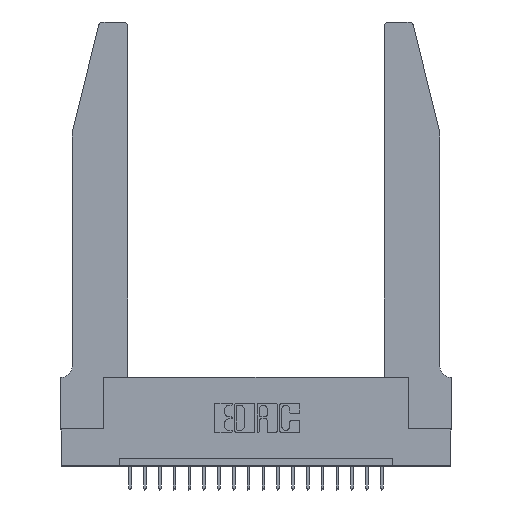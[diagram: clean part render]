
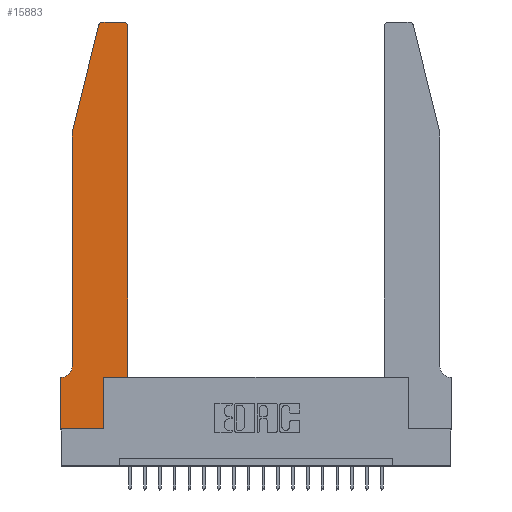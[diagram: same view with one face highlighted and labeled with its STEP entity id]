
A CAD part, top view. The second image highlights one B-rep face of the part: STEP entity #15883.
In plain terms, the highlighted planar face has unit normal (0, 0, 1).
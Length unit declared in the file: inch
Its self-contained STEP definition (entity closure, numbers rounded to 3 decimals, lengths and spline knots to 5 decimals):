
#17 = VECTOR ( 'NONE', #19088, 39.37008 ) ;
#201 = DIRECTION ( 'NONE',  ( -1., 0., 0. ) ) ;
#575 = ORIENTED_EDGE ( 'NONE', *, *, #8515, .T. ) ;
#639 = CARTESIAN_POINT ( 'NONE',  ( 0.4205, 2.75, 0.37 ) ) ;
#790 = DIRECTION ( 'NONE',  ( 0., 1., 0. ) ) ;
#1388 = EDGE_CURVE ( 'NONE', #5708, #19935, #13388, .T. ) ;
#1568 = ORIENTED_EDGE ( 'NONE', *, *, #12442, .T. ) ;
#1596 = DIRECTION ( 'NONE',  ( 1., 0., 0. ) ) ;
#1739 = DIRECTION ( 'NONE',  ( 1., 0., 0. ) ) ;
#1808 = EDGE_CURVE ( 'NONE', #3204, #11223, #20917, .T. ) ;
#1840 = EDGE_CURVE ( 'NONE', #6400, #2131, #21188, .T. ) ;
#1881 = EDGE_CURVE ( 'NONE', #11223, #20557, #5774, .T. ) ;
#1903 = VECTOR ( 'NONE', #7939, 39.37008 ) ;
#2131 = VERTEX_POINT ( 'NONE', #10437 ) ;
#2134 = DIRECTION ( 'NONE',  ( 1., 0., 0. ) ) ;
#2150 = CARTESIAN_POINT ( 'NONE',  ( 0.2865, 0.35, 0.37 ) ) ;
#2797 = VECTOR ( 'NONE', #13358, 39.37008 ) ;
#2940 = LINE ( 'NONE', #2150, #15995 ) ;
#2977 = ORIENTED_EDGE ( 'NONE', *, *, #1881, .T. ) ;
#3045 = ORIENTED_EDGE ( 'NONE', *, *, #10656, .T. ) ;
#3204 = VERTEX_POINT ( 'NONE', #639 ) ;
#3388 = LINE ( 'NONE', #4214, #17 ) ;
#3402 = ORIENTED_EDGE ( 'NONE', *, *, #15248, .T. ) ;
#3446 = ORIENTED_EDGE ( 'NONE', *, *, #16910, .T. ) ;
#3575 = CARTESIAN_POINT ( 'NONE',  ( 0.0755, 2., 0.37 ) ) ;
#3638 = DIRECTION ( 'NONE',  ( -1., 0., 0. ) ) ;
#3684 = CARTESIAN_POINT ( 'NONE',  ( 0.284, 2.72, 0.37 ) ) ;
#3869 = CARTESIAN_POINT ( 'NONE',  ( 0.0055, 0.35, 0.37 ) ) ;
#3877 = DIRECTION ( 'NONE',  ( 0., 0., 1. ) ) ;
#4214 = CARTESIAN_POINT ( 'NONE',  ( 0.4505, 0.35, 0.37 ) ) ;
#4761 = DIRECTION ( 'NONE',  ( 1., 0., 0. ) ) ;
#5011 = DIRECTION ( 'NONE',  ( -1., 0., 0. ) ) ;
#5015 = CARTESIAN_POINT ( 'NONE',  ( 0.0755, 2., 0.37 ) ) ;
#5204 = CARTESIAN_POINT ( 'NONE',  ( 0.4505, 2.72, 0.37 ) ) ;
#5616 = CIRCLE ( 'NONE', #18930, 0.03 ) ;
#5708 = VERTEX_POINT ( 'NONE', #9108 ) ;
#5774 = CIRCLE ( 'NONE', #16114, 0.03 ) ;
#6172 = EDGE_CURVE ( 'NONE', #19386, #3204, #5616, .T. ) ;
#6400 = VERTEX_POINT ( 'NONE', #20015 ) ;
#6699 = CARTESIAN_POINT ( 'NONE',  ( 0., 0., 0.37 ) ) ;
#6913 = CARTESIAN_POINT ( 'NONE',  ( 0.25487, 2.72718, 0.37 ) ) ;
#7939 = DIRECTION ( 'NONE',  ( -0.239, -0.971, 0. ) ) ;
#8505 = ORIENTED_EDGE ( 'NONE', *, *, #19417, .T. ) ;
#8515 = EDGE_CURVE ( 'NONE', #15281, #6400, #2940, .T. ) ;
#8684 = ORIENTED_EDGE ( 'NONE', *, *, #1388, .T. ) ;
#8704 = CARTESIAN_POINT ( 'NONE',  ( 0.0755, 0.35, 0.37 ) ) ;
#8760 = CARTESIAN_POINT ( 'NONE',  ( 0.4205, 2.72, 0.37 ) ) ;
#8898 = DIRECTION ( 'NONE',  ( 0., 0., -1. ) ) ;
#9108 = CARTESIAN_POINT ( 'NONE',  ( 0.0755, 0.42, 0.37 ) ) ;
#9247 = VERTEX_POINT ( 'NONE', #16477 ) ;
#9501 = DIRECTION ( 'NONE',  ( 0., 0., 1. ) ) ;
#9947 = VECTOR ( 'NONE', #5011, 39.37008 ) ;
#10172 = AXIS2_PLACEMENT_3D ( 'NONE', #13110, #9501, #4761 ) ;
#10437 = CARTESIAN_POINT ( 'NONE',  ( 0.4505, 0.35, 0.37 ) ) ;
#10559 = FACE_OUTER_BOUND ( 'NONE', #17041, .T. ) ;
#10656 = EDGE_CURVE ( 'NONE', #2131, #19386, #3388, .T. ) ;
#11223 = VERTEX_POINT ( 'NONE', #12341 ) ;
#11226 = CARTESIAN_POINT ( 'NONE',  ( 0.2865, 0., 0.37 ) ) ;
#12341 = CARTESIAN_POINT ( 'NONE',  ( 0.284, 2.75, 0.37 ) ) ;
#12442 = EDGE_CURVE ( 'NONE', #9247, #15281, #13769, .T. ) ;
#12473 = AXIS2_PLACEMENT_3D ( 'NONE', #15330, #8898, #3638 ) ;
#12621 = CARTESIAN_POINT ( 'NONE',  ( 0.0755, 2., 0.37 ) ) ;
#12951 = LINE ( 'NONE', #12621, #16333 ) ;
#12958 = CARTESIAN_POINT ( 'NONE',  ( 0., 0., 0.37 ) ) ;
#13110 = CARTESIAN_POINT ( 'NONE',  ( 0., 0.35, 0.37 ) ) ;
#13222 = CARTESIAN_POINT ( 'NONE',  ( 0.4505, 0.35, 0.37 ) ) ;
#13358 = DIRECTION ( 'NONE',  ( 0., -1., 0. ) ) ;
#13388 = CIRCLE ( 'NONE', #12473, 0.07 ) ;
#13651 = ORIENTED_EDGE ( 'NONE', *, *, #1840, .T. ) ;
#13769 = LINE ( 'NONE', #12958, #14058 ) ;
#14039 = LINE ( 'NONE', #6699, #2797 ) ;
#14058 = VECTOR ( 'NONE', #21166, 39.37008 ) ;
#14067 = ORIENTED_EDGE ( 'NONE', *, *, #20457, .T. ) ;
#14738 = LINE ( 'NONE', #3575, #1903 ) ;
#15042 = CARTESIAN_POINT ( 'NONE',  ( 0.2605, 2.75, 0.37 ) ) ;
#15169 = DIRECTION ( 'NONE',  ( 0., 0., 1. ) ) ;
#15248 = EDGE_CURVE ( 'NONE', #18689, #5708, #12951, .T. ) ;
#15281 = VERTEX_POINT ( 'NONE', #11226 ) ;
#15330 = CARTESIAN_POINT ( 'NONE',  ( 0.0055, 0.42, 0.37 ) ) ;
#15602 = ORIENTED_EDGE ( 'NONE', *, *, #1808, .T. ) ;
#15883 = ADVANCED_FACE ( 'NONE', ( #10559 ), #21183, .T. ) ;
#15995 = VECTOR ( 'NONE', #790, 39.37008 ) ;
#16114 = AXIS2_PLACEMENT_3D ( 'NONE', #3684, #15169, #1739 ) ;
#16333 = VECTOR ( 'NONE', #20777, 39.37008 ) ;
#16477 = CARTESIAN_POINT ( 'NONE',  ( 0., 0., 0.37 ) ) ;
#16761 = VECTOR ( 'NONE', #1596, 39.37008 ) ;
#16910 = EDGE_CURVE ( 'NONE', #20557, #18689, #14738, .T. ) ;
#17041 = EDGE_LOOP ( 'NONE', ( #15602, #2977, #3446, #3402, #8684, #8505, #14067, #1568, #575, #13651, #3045, #18077 ) ) ;
#18077 = ORIENTED_EDGE ( 'NONE', *, *, #6172, .T. ) ;
#18689 = VERTEX_POINT ( 'NONE', #5015 ) ;
#18744 = LINE ( 'NONE', #8704, #21626 ) ;
#18930 = AXIS2_PLACEMENT_3D ( 'NONE', #8760, #3877, #2134 ) ;
#18964 = CARTESIAN_POINT ( 'NONE',  ( 0., 0.35, 0.37 ) ) ;
#19088 = DIRECTION ( 'NONE',  ( 0., 1., 0. ) ) ;
#19386 = VERTEX_POINT ( 'NONE', #5204 ) ;
#19417 = EDGE_CURVE ( 'NONE', #19935, #20054, #18744, .T. ) ;
#19935 = VERTEX_POINT ( 'NONE', #3869 ) ;
#20015 = CARTESIAN_POINT ( 'NONE',  ( 0.2865, 0.35, 0.37 ) ) ;
#20054 = VERTEX_POINT ( 'NONE', #18964 ) ;
#20457 = EDGE_CURVE ( 'NONE', #20054, #9247, #14039, .T. ) ;
#20557 = VERTEX_POINT ( 'NONE', #6913 ) ;
#20777 = DIRECTION ( 'NONE',  ( 0., -1., 0. ) ) ;
#20917 = LINE ( 'NONE', #15042, #9947 ) ;
#21166 = DIRECTION ( 'NONE',  ( 1., 0., 0. ) ) ;
#21183 = PLANE ( 'NONE',  #10172 ) ;
#21188 = LINE ( 'NONE', #13222, #16761 ) ;
#21626 = VECTOR ( 'NONE', #201, 39.37008 ) ;
